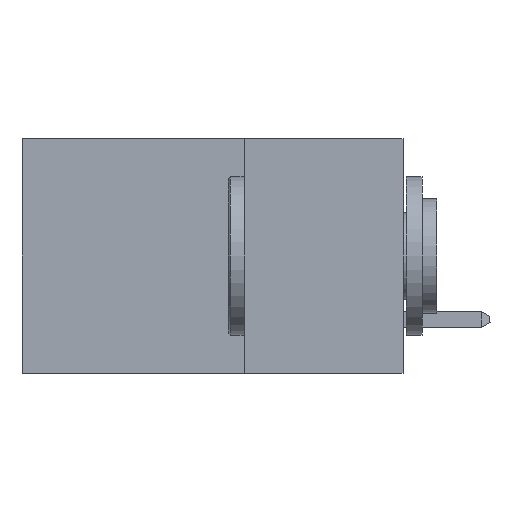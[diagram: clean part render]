
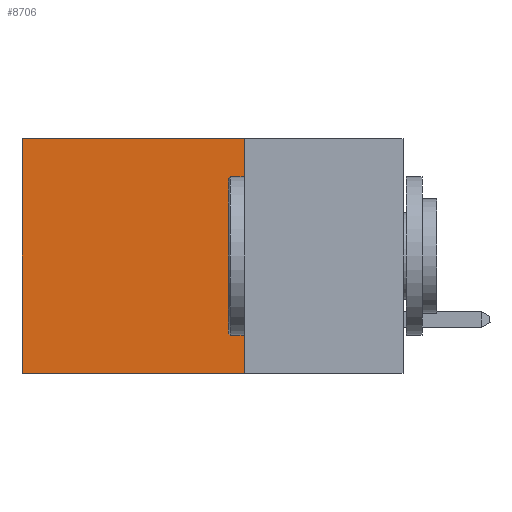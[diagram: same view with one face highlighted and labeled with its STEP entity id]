
A CAD part, left-side view. The second image highlights one B-rep face of the part: STEP entity #8706.
In plain terms, the highlighted planar face has unit normal (-1, 0, 0).
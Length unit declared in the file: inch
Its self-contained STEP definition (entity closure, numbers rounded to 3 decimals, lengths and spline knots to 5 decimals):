
#734 = VERTEX_POINT ( 'NONE', #17906 ) ;
#1028 = VERTEX_POINT ( 'NONE', #14221 ) ;
#1770 = LINE ( 'NONE', #12076, #18170 ) ;
#1982 = ORIENTED_EDGE ( 'NONE', *, *, #10149, .T. ) ;
#2622 = ORIENTED_EDGE ( 'NONE', *, *, #6100, .F. ) ;
#3269 = LINE ( 'NONE', #8413, #27769 ) ;
#4099 = VECTOR ( 'NONE', #28954, 39.37008 ) ;
#4449 = CARTESIAN_POINT ( 'NONE',  ( 0.2875, 0.6, 0. ) ) ;
#4606 = DIRECTION ( 'NONE',  ( 0., 1., 0. ) ) ;
#5850 = EDGE_LOOP ( 'NONE', ( #1982, #8873, #2622, #21272 ) ) ;
#6100 = EDGE_CURVE ( 'NONE', #27708, #734, #8537, .T. ) ;
#6987 = VECTOR ( 'NONE', #28081, 39.37008 ) ;
#7808 = CARTESIAN_POINT ( 'NONE',  ( 0.2875, 0.6, -0.37 ) ) ;
#8413 = CARTESIAN_POINT ( 'NONE',  ( 0.2875, 0.25, 0. ) ) ;
#8537 = LINE ( 'NONE', #10654, #6987 ) ;
#8706 = ADVANCED_FACE ( 'NONE', ( #30190 ), #27856, .F. ) ;
#8873 = ORIENTED_EDGE ( 'NONE', *, *, #17107, .F. ) ;
#10149 = EDGE_CURVE ( 'NONE', #1028, #18917, #23585, .T. ) ;
#10654 = CARTESIAN_POINT ( 'NONE',  ( 0.2875, 0.25, 0. ) ) ;
#12076 = CARTESIAN_POINT ( 'NONE',  ( 0.2875, 0.25, -0.37 ) ) ;
#14221 = CARTESIAN_POINT ( 'NONE',  ( 0.2875, 0.6, 0. ) ) ;
#17107 = EDGE_CURVE ( 'NONE', #734, #18917, #1770, .T. ) ;
#17199 = EDGE_CURVE ( 'NONE', #27708, #1028, #3269, .T. ) ;
#17906 = CARTESIAN_POINT ( 'NONE',  ( 0.2875, 0.25, -0.37 ) ) ;
#18170 = VECTOR ( 'NONE', #24308, 39.37008 ) ;
#18917 = VERTEX_POINT ( 'NONE', #7808 ) ;
#20661 = CARTESIAN_POINT ( 'NONE',  ( 0.2875, 0.25, 0. ) ) ;
#21272 = ORIENTED_EDGE ( 'NONE', *, *, #17199, .T. ) ;
#23585 = LINE ( 'NONE', #4449, #4099 ) ;
#23859 = CARTESIAN_POINT ( 'NONE',  ( 0.2875, 0.25, 0. ) ) ;
#24308 = DIRECTION ( 'NONE',  ( 0., 1., 0. ) ) ;
#25485 = AXIS2_PLACEMENT_3D ( 'NONE', #20661, #29978, #30306 ) ;
#27708 = VERTEX_POINT ( 'NONE', #23859 ) ;
#27769 = VECTOR ( 'NONE', #4606, 39.37008 ) ;
#27856 = PLANE ( 'NONE',  #25485 ) ;
#28081 = DIRECTION ( 'NONE',  ( 0., 0., -1. ) ) ;
#28954 = DIRECTION ( 'NONE',  ( 0., 0., -1. ) ) ;
#29978 = DIRECTION ( 'NONE',  ( 1., 0., 0. ) ) ;
#30190 = FACE_OUTER_BOUND ( 'NONE', #5850, .T. ) ;
#30306 = DIRECTION ( 'NONE',  ( 0., 0., -1. ) ) ;
